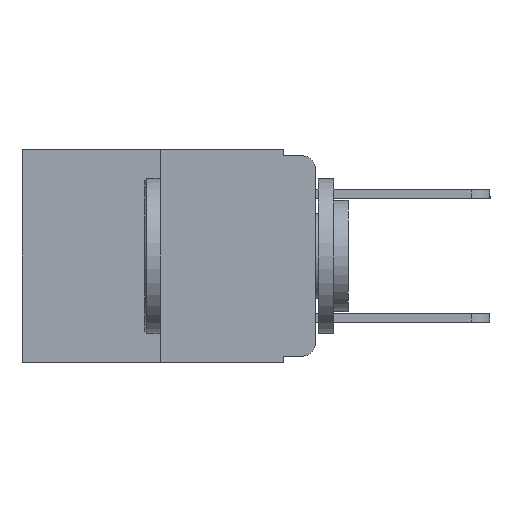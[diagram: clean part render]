
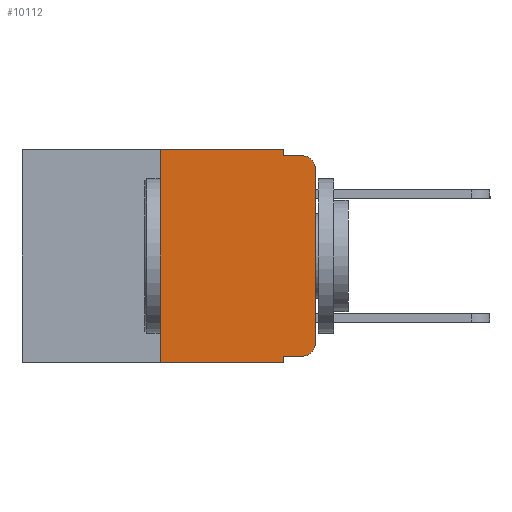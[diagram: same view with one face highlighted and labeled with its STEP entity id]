
A CAD part, left-side view. The second image highlights one B-rep face of the part: STEP entity #10112.
In plain terms, the highlighted planar face has unit normal (-1, 0, 0).
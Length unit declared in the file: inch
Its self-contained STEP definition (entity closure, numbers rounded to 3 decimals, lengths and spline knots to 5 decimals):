
#68 = VERTEX_POINT ( 'NONE', #9966 ) ;
#92 = CARTESIAN_POINT ( 'NONE',  ( 0., 0., 0. ) ) ;
#136 = EDGE_CURVE ( 'NONE', #1088, #5593, #808, .T. ) ;
#239 = DIRECTION ( 'NONE',  ( 0., 0., 1. ) ) ;
#464 = DIRECTION ( 'NONE',  ( 0., 0., -1. ) ) ;
#569 = DIRECTION ( 'NONE',  ( 0., 0., -1. ) ) ;
#808 = LINE ( 'NONE', #3101, #11708 ) ;
#810 = VERTEX_POINT ( 'NONE', #5877 ) ;
#822 = DIRECTION ( 'NONE',  ( 0., 0., 1. ) ) ;
#830 = VERTEX_POINT ( 'NONE', #5994 ) ;
#1088 = VERTEX_POINT ( 'NONE', #5727 ) ;
#1822 = EDGE_LOOP ( 'NONE', ( #3441, #4182, #8394, #6301, #6784, #6754, #8008, #7662, #8370, #7886 ) ) ;
#2127 = PLANE ( 'NONE',  #10595 ) ;
#2647 = LINE ( 'NONE', #9902, #12985 ) ;
#2711 = EDGE_CURVE ( 'NONE', #9074, #6098, #9112, .T. ) ;
#2900 = CARTESIAN_POINT ( 'NONE',  ( 0., 0.051, -0.343 ) ) ;
#3033 = AXIS2_PLACEMENT_3D ( 'NONE', #13010, #7313, #569 ) ;
#3101 = CARTESIAN_POINT ( 'NONE',  ( 0., 0.051, -0.333 ) ) ;
#3114 = CARTESIAN_POINT ( 'NONE',  ( 0., 0.25, 0. ) ) ;
#3132 = DIRECTION ( 'NONE',  ( 0., -1., 0. ) ) ;
#3175 = EDGE_CURVE ( 'NONE', #830, #5186, #6334, .T. ) ;
#3191 = LINE ( 'NONE', #13433, #13380 ) ;
#3366 = DIRECTION ( 'NONE',  ( 1., 0., 0. ) ) ;
#3441 = ORIENTED_EDGE ( 'NONE', *, *, #5305, .T. ) ;
#3684 = EDGE_CURVE ( 'NONE', #9496, #810, #10764, .T. ) ;
#3797 = EDGE_CURVE ( 'NONE', #830, #7455, #6619, .T. ) ;
#4182 = ORIENTED_EDGE ( 'NONE', *, *, #3684, .T. ) ;
#4653 = VECTOR ( 'NONE', #12313, 39.37008 ) ;
#5016 = CARTESIAN_POINT ( 'NONE',  ( 0., 0.473, -0.343 ) ) ;
#5186 = VERTEX_POINT ( 'NONE', #2900 ) ;
#5305 = EDGE_CURVE ( 'NONE', #68, #9496, #10741, .T. ) ;
#5324 = CARTESIAN_POINT ( 'NONE',  ( 0., 0.051, 0. ) ) ;
#5593 = VERTEX_POINT ( 'NONE', #9811 ) ;
#5727 = CARTESIAN_POINT ( 'NONE',  ( 0., 0.051, -0.333 ) ) ;
#5877 = CARTESIAN_POINT ( 'NONE',  ( 0., 0.02, -0.01 ) ) ;
#5994 = CARTESIAN_POINT ( 'NONE',  ( 0., 0.25, -0.343 ) ) ;
#5999 = VECTOR ( 'NONE', #8051, 39.37008 ) ;
#6098 = VERTEX_POINT ( 'NONE', #9281 ) ;
#6120 = EDGE_CURVE ( 'NONE', #1088, #5186, #2647, .T. ) ;
#6301 = ORIENTED_EDGE ( 'NONE', *, *, #2711, .F. ) ;
#6334 = LINE ( 'NONE', #5016, #5999 ) ;
#6379 = EDGE_CURVE ( 'NONE', #6098, #810, #3191, .T. ) ;
#6544 = CARTESIAN_POINT ( 'NONE',  ( 0., 0.02, -0.03 ) ) ;
#6619 = LINE ( 'NONE', #3114, #11763 ) ;
#6754 = ORIENTED_EDGE ( 'NONE', *, *, #3797, .F. ) ;
#6784 = ORIENTED_EDGE ( 'NONE', *, *, #8919, .F. ) ;
#6997 = CIRCLE ( 'NONE', #3033, 0.02 ) ;
#7313 = DIRECTION ( 'NONE',  ( -1., 0., 0. ) ) ;
#7430 = VECTOR ( 'NONE', #12916, 39.37008 ) ;
#7455 = VERTEX_POINT ( 'NONE', #9765 ) ;
#7662 = ORIENTED_EDGE ( 'NONE', *, *, #6120, .F. ) ;
#7724 = FACE_OUTER_BOUND ( 'NONE', #1822, .T. ) ;
#7737 = DIRECTION ( 'NONE',  ( 0., 0., -1. ) ) ;
#7886 = ORIENTED_EDGE ( 'NONE', *, *, #9924, .T. ) ;
#8008 = ORIENTED_EDGE ( 'NONE', *, *, #3175, .T. ) ;
#8051 = DIRECTION ( 'NONE',  ( 0., -1., 0. ) ) ;
#8087 = LINE ( 'NONE', #9180, #7430 ) ;
#8370 = ORIENTED_EDGE ( 'NONE', *, *, #136, .T. ) ;
#8394 = ORIENTED_EDGE ( 'NONE', *, *, #6379, .F. ) ;
#8400 = CARTESIAN_POINT ( 'NONE',  ( 0., 0.051, 0. ) ) ;
#8919 = EDGE_CURVE ( 'NONE', #7455, #9074, #8087, .T. ) ;
#9074 = VERTEX_POINT ( 'NONE', #5324 ) ;
#9112 = LINE ( 'NONE', #8400, #4653 ) ;
#9180 = CARTESIAN_POINT ( 'NONE',  ( 0., 0.473, 0. ) ) ;
#9281 = CARTESIAN_POINT ( 'NONE',  ( 0., 0.051, -0.01 ) ) ;
#9485 = CARTESIAN_POINT ( 'NONE',  ( 0., 0.473, 0. ) ) ;
#9496 = VERTEX_POINT ( 'NONE', #9794 ) ;
#9552 = AXIS2_PLACEMENT_3D ( 'NONE', #6544, #11243, #464 ) ;
#9765 = CARTESIAN_POINT ( 'NONE',  ( 0., 0.25, 0. ) ) ;
#9794 = CARTESIAN_POINT ( 'NONE',  ( 0., 0., -0.03 ) ) ;
#9811 = CARTESIAN_POINT ( 'NONE',  ( 0., 0.02, -0.333 ) ) ;
#9902 = CARTESIAN_POINT ( 'NONE',  ( 0., 0.051, 0. ) ) ;
#9924 = EDGE_CURVE ( 'NONE', #5593, #68, #6997, .T. ) ;
#9966 = CARTESIAN_POINT ( 'NONE',  ( 0., 0., -0.313 ) ) ;
#10112 = ADVANCED_FACE ( 'NONE', ( #7724 ), #2127, .F. ) ;
#10509 = DIRECTION ( 'NONE',  ( 0., 0., -1. ) ) ;
#10595 = AXIS2_PLACEMENT_3D ( 'NONE', #9485, #3366, #10509 ) ;
#10741 = LINE ( 'NONE', #92, #11022 ) ;
#10764 = CIRCLE ( 'NONE', #9552, 0.02 ) ;
#11022 = VECTOR ( 'NONE', #239, 39.37008 ) ;
#11243 = DIRECTION ( 'NONE',  ( -1., 0., 0. ) ) ;
#11708 = VECTOR ( 'NONE', #3132, 39.37008 ) ;
#11763 = VECTOR ( 'NONE', #822, 39.37008 ) ;
#12313 = DIRECTION ( 'NONE',  ( 0., 0., -1. ) ) ;
#12916 = DIRECTION ( 'NONE',  ( 0., -1., 0. ) ) ;
#12985 = VECTOR ( 'NONE', #7737, 39.37008 ) ;
#13010 = CARTESIAN_POINT ( 'NONE',  ( 0., 0.02, -0.313 ) ) ;
#13055 = DIRECTION ( 'NONE',  ( 0., -1., 0. ) ) ;
#13380 = VECTOR ( 'NONE', #13055, 39.37008 ) ;
#13433 = CARTESIAN_POINT ( 'NONE',  ( 0., 0.051, -0.01 ) ) ;
